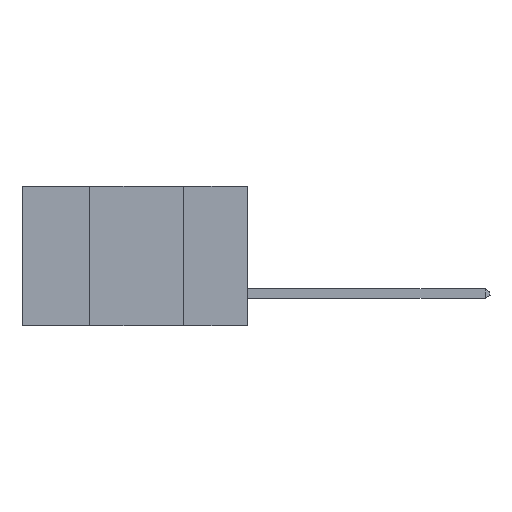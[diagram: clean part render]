
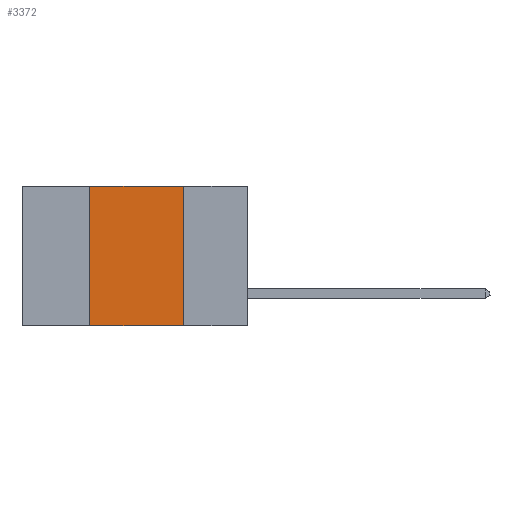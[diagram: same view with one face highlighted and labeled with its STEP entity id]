
A CAD part, left-side view. The second image highlights one B-rep face of the part: STEP entity #3372.
In plain terms, the highlighted planar face has unit normal (-1, 0, 0).
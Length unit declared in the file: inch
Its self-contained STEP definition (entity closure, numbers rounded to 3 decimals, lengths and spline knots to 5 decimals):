
#258 = DIRECTION ( 'NONE',  ( 0., 0., -1. ) ) ;
#699 = LINE ( 'NONE', #8870, #5585 ) ;
#752 = DIRECTION ( 'NONE',  ( 1., 0., 0. ) ) ;
#756 = DIRECTION ( 'NONE',  ( 0., -1., 0. ) ) ;
#1002 = CARTESIAN_POINT ( 'NONE',  ( 0., 0.6, 0. ) ) ;
#2312 = DIRECTION ( 'NONE',  ( 0., -1., 0. ) ) ;
#3372 = ADVANCED_FACE ( 'NONE', ( #9853 ), #11541, .F. ) ;
#4457 = CARTESIAN_POINT ( 'NONE',  ( 0., 0.42, -0.37 ) ) ;
#4986 = EDGE_CURVE ( 'NONE', #9786, #17060, #12762, .T. ) ;
#5261 = ORIENTED_EDGE ( 'NONE', *, *, #4986, .F. ) ;
#5585 = VECTOR ( 'NONE', #2312, 39.37008 ) ;
#5769 = EDGE_LOOP ( 'NONE', ( #5261, #17745, #14311, #14162 ) ) ;
#5952 = VERTEX_POINT ( 'NONE', #4457 ) ;
#6407 = EDGE_CURVE ( 'NONE', #15347, #9786, #12065, .T. ) ;
#6487 = EDGE_CURVE ( 'NONE', #5952, #17060, #699, .T. ) ;
#6950 = AXIS2_PLACEMENT_3D ( 'NONE', #13184, #752, #7016 ) ;
#7016 = DIRECTION ( 'NONE',  ( 0., 0., -1. ) ) ;
#8738 = DIRECTION ( 'NONE',  ( 0., 0., 1. ) ) ;
#8870 = CARTESIAN_POINT ( 'NONE',  ( 0., 0.6, -0.37 ) ) ;
#9786 = VERTEX_POINT ( 'NONE', #12149 ) ;
#9853 = FACE_OUTER_BOUND ( 'NONE', #5769, .T. ) ;
#10338 = VECTOR ( 'NONE', #8738, 39.37008 ) ;
#11541 = PLANE ( 'NONE',  #6950 ) ;
#12065 = LINE ( 'NONE', #1002, #17714 ) ;
#12149 = CARTESIAN_POINT ( 'NONE',  ( 0., 0.17, 0. ) ) ;
#12762 = LINE ( 'NONE', #18967, #19583 ) ;
#13184 = CARTESIAN_POINT ( 'NONE',  ( 0., 0.6, 0. ) ) ;
#13252 = CARTESIAN_POINT ( 'NONE',  ( 0., 0.42, 0. ) ) ;
#14002 = LINE ( 'NONE', #13252, #10338 ) ;
#14162 = ORIENTED_EDGE ( 'NONE', *, *, #6487, .T. ) ;
#14311 = ORIENTED_EDGE ( 'NONE', *, *, #16403, .F. ) ;
#15347 = VERTEX_POINT ( 'NONE', #18492 ) ;
#16403 = EDGE_CURVE ( 'NONE', #5952, #15347, #14002, .T. ) ;
#16875 = CARTESIAN_POINT ( 'NONE',  ( 0., 0.17, -0.37 ) ) ;
#17060 = VERTEX_POINT ( 'NONE', #16875 ) ;
#17714 = VECTOR ( 'NONE', #756, 39.37008 ) ;
#17745 = ORIENTED_EDGE ( 'NONE', *, *, #6407, .F. ) ;
#18492 = CARTESIAN_POINT ( 'NONE',  ( 0., 0.42, 0. ) ) ;
#18967 = CARTESIAN_POINT ( 'NONE',  ( 0., 0.17, 0. ) ) ;
#19583 = VECTOR ( 'NONE', #258, 39.37008 ) ;
